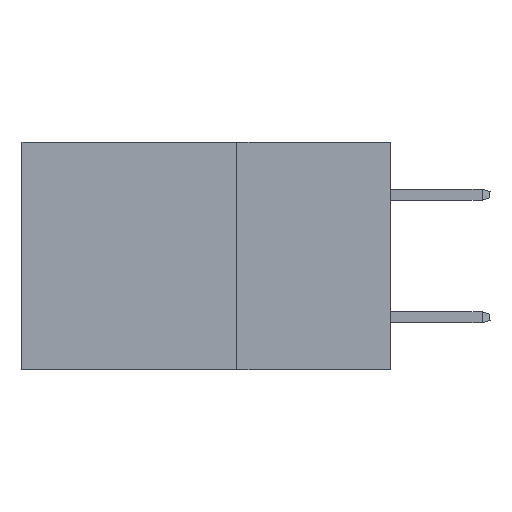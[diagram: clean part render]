
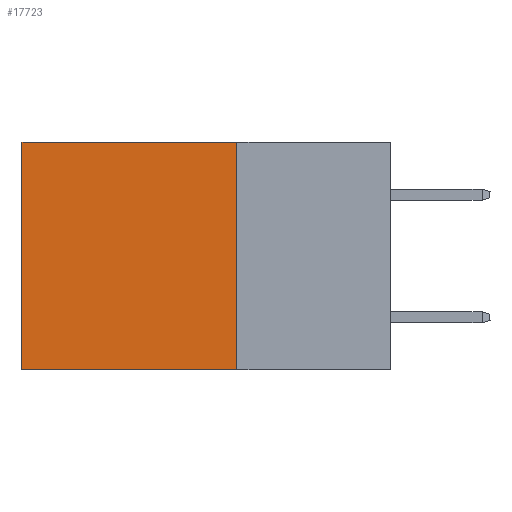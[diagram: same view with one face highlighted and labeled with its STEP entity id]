
A CAD part, left-side view. The second image highlights one B-rep face of the part: STEP entity #17723.
In plain terms, the highlighted planar face has unit normal (-1, 0, 0).
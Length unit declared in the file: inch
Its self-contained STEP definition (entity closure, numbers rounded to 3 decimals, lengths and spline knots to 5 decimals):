
#295 = VECTOR ( 'NONE', #6289, 39.37008 ) ;
#437 = PLANE ( 'NONE',  #11336 ) ;
#900 = CARTESIAN_POINT ( 'NONE',  ( 0.2875, 0.25, 0. ) ) ;
#2051 = CARTESIAN_POINT ( 'NONE',  ( 0.2875, 0.6, 0. ) ) ;
#2321 = CARTESIAN_POINT ( 'NONE',  ( 0.2875, 0.25, 0. ) ) ;
#3778 = CARTESIAN_POINT ( 'NONE',  ( 0.2875, 0.25, 0. ) ) ;
#4079 = CARTESIAN_POINT ( 'NONE',  ( 0.2875, 0.25, -0.37 ) ) ;
#5474 = FACE_OUTER_BOUND ( 'NONE', #15024, .T. ) ;
#6289 = DIRECTION ( 'NONE',  ( 0., 0., -1. ) ) ;
#6333 = EDGE_CURVE ( 'NONE', #11994, #19084, #11568, .T. ) ;
#6894 = VECTOR ( 'NONE', #18730, 39.37008 ) ;
#6976 = ORIENTED_EDGE ( 'NONE', *, *, #6333, .T. ) ;
#7911 = DIRECTION ( 'NONE',  ( 0., 1., 0. ) ) ;
#11336 = AXIS2_PLACEMENT_3D ( 'NONE', #2321, #19510, #15120 ) ;
#11568 = LINE ( 'NONE', #2051, #295 ) ;
#11716 = LINE ( 'NONE', #900, #22175 ) ;
#11994 = VERTEX_POINT ( 'NONE', #25091 ) ;
#14373 = EDGE_CURVE ( 'NONE', #17775, #11994, #11716, .T. ) ;
#14476 = LINE ( 'NONE', #14895, #6894 ) ;
#14895 = CARTESIAN_POINT ( 'NONE',  ( 0.2875, 0.25, -0.37 ) ) ;
#14957 = VERTEX_POINT ( 'NONE', #4079 ) ;
#15024 = EDGE_LOOP ( 'NONE', ( #6976, #18202, #26308, #15322 ) ) ;
#15120 = DIRECTION ( 'NONE',  ( 0., 0., -1. ) ) ;
#15322 = ORIENTED_EDGE ( 'NONE', *, *, #14373, .T. ) ;
#15657 = DIRECTION ( 'NONE',  ( 0., 0., -1. ) ) ;
#15977 = EDGE_CURVE ( 'NONE', #17775, #14957, #26896, .T. ) ;
#17723 = ADVANCED_FACE ( 'NONE', ( #5474 ), #437, .F. ) ;
#17775 = VERTEX_POINT ( 'NONE', #21518 ) ;
#18202 = ORIENTED_EDGE ( 'NONE', *, *, #23312, .F. ) ;
#18730 = DIRECTION ( 'NONE',  ( 0., 1., 0. ) ) ;
#19084 = VERTEX_POINT ( 'NONE', #24188 ) ;
#19510 = DIRECTION ( 'NONE',  ( 1., 0., 0. ) ) ;
#20704 = VECTOR ( 'NONE', #15657, 39.37008 ) ;
#21518 = CARTESIAN_POINT ( 'NONE',  ( 0.2875, 0.25, 0. ) ) ;
#22175 = VECTOR ( 'NONE', #7911, 39.37008 ) ;
#23312 = EDGE_CURVE ( 'NONE', #14957, #19084, #14476, .T. ) ;
#24188 = CARTESIAN_POINT ( 'NONE',  ( 0.2875, 0.6, -0.37 ) ) ;
#25091 = CARTESIAN_POINT ( 'NONE',  ( 0.2875, 0.6, 0. ) ) ;
#26308 = ORIENTED_EDGE ( 'NONE', *, *, #15977, .F. ) ;
#26896 = LINE ( 'NONE', #3778, #20704 ) ;
